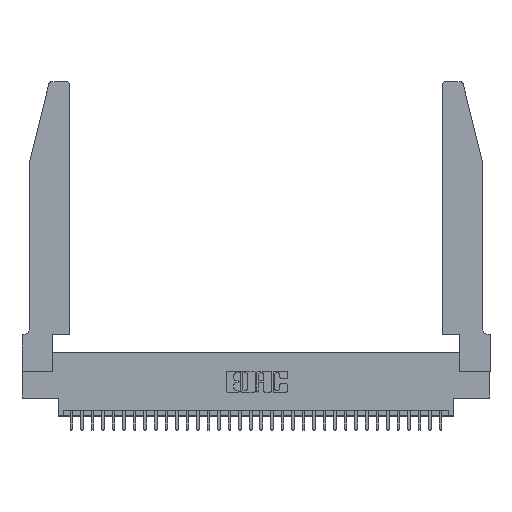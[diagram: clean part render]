
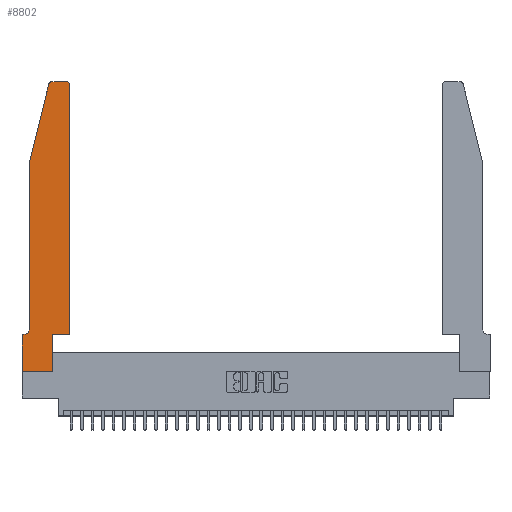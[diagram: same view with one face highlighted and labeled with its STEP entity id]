
A CAD part, top view. The second image highlights one B-rep face of the part: STEP entity #8802.
In plain terms, the highlighted planar face has unit normal (0, 0, 1).
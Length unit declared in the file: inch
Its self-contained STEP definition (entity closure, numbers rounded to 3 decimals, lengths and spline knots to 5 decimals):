
#25 = VERTEX_POINT ( 'NONE', #307 ) ;
#42 = CARTESIAN_POINT ( 'NONE',  ( 0.4505, 2.72, 0.37 ) ) ;
#307 = CARTESIAN_POINT ( 'NONE',  ( 0.0755, 0.42, 0.37 ) ) ;
#499 = CARTESIAN_POINT ( 'NONE',  ( 0.2865, 0.35, 0.37 ) ) ;
#1762 = VERTEX_POINT ( 'NONE', #8056 ) ;
#1792 = DIRECTION ( 'NONE',  ( 1., 0., 0. ) ) ;
#1813 = ORIENTED_EDGE ( 'NONE', *, *, #8376, .T. ) ;
#1943 = DIRECTION ( 'NONE',  ( 1., 0., 0. ) ) ;
#2092 = DIRECTION ( 'NONE',  ( 0., 0., -1. ) ) ;
#2441 = VECTOR ( 'NONE', #3148, 39.37008 ) ;
#2450 = DIRECTION ( 'NONE',  ( 1., 0., 0. ) ) ;
#2932 = LINE ( 'NONE', #30753, #23141 ) ;
#3148 = DIRECTION ( 'NONE',  ( 0., 1., 0. ) ) ;
#3216 = CARTESIAN_POINT ( 'NONE',  ( 0.4205, 2.75, 0.37 ) ) ;
#3739 = EDGE_CURVE ( 'NONE', #6368, #6413, #22148, .T. ) ;
#3926 = EDGE_CURVE ( 'NONE', #12568, #24901, #11070, .T. ) ;
#4892 = CARTESIAN_POINT ( 'NONE',  ( 0., 0., 0.37 ) ) ;
#4934 = VECTOR ( 'NONE', #24225, 39.37008 ) ;
#5141 = CARTESIAN_POINT ( 'NONE',  ( 0.4505, 0.35, 0.37 ) ) ;
#5718 = VERTEX_POINT ( 'NONE', #18212 ) ;
#6053 = DIRECTION ( 'NONE',  ( 0., -1., 0. ) ) ;
#6120 = ORIENTED_EDGE ( 'NONE', *, *, #23613, .T. ) ;
#6368 = VERTEX_POINT ( 'NONE', #12994 ) ;
#6413 = VERTEX_POINT ( 'NONE', #42 ) ;
#6601 = ORIENTED_EDGE ( 'NONE', *, *, #31092, .T. ) ;
#7410 = CARTESIAN_POINT ( 'NONE',  ( 0.0755, 0.35, 0.37 ) ) ;
#7532 = DIRECTION ( 'NONE',  ( -1., 0., 0. ) ) ;
#8056 = CARTESIAN_POINT ( 'NONE',  ( 0.0055, 0.35, 0.37 ) ) ;
#8376 = EDGE_CURVE ( 'NONE', #21702, #12568, #32842, .T. ) ;
#8802 = ADVANCED_FACE ( 'NONE', ( #28333 ), #31266, .T. ) ;
#9107 = ORIENTED_EDGE ( 'NONE', *, *, #26627, .T. ) ;
#9505 = CARTESIAN_POINT ( 'NONE',  ( 0., 0., 0.37 ) ) ;
#9605 = CARTESIAN_POINT ( 'NONE',  ( 0.284, 2.75, 0.37 ) ) ;
#10192 = EDGE_CURVE ( 'NONE', #20287, #16153, #25273, .T. ) ;
#10235 = LINE ( 'NONE', #4892, #24139 ) ;
#11070 = CIRCLE ( 'NONE', #30890, 0.03 ) ;
#11318 = CARTESIAN_POINT ( 'NONE',  ( 0.2605, 2.75, 0.37 ) ) ;
#12568 = VERTEX_POINT ( 'NONE', #9605 ) ;
#12684 = CIRCLE ( 'NONE', #32647, 0.07 ) ;
#12994 = CARTESIAN_POINT ( 'NONE',  ( 0.4505, 0.35, 0.37 ) ) ;
#13008 = EDGE_CURVE ( 'NONE', #5718, #25, #16957, .T. ) ;
#13115 = DIRECTION ( 'NONE',  ( 0., 1., 0. ) ) ;
#13818 = LINE ( 'NONE', #7410, #32206 ) ;
#14341 = VECTOR ( 'NONE', #13115, 39.37008 ) ;
#14389 = CARTESIAN_POINT ( 'NONE',  ( 0.284, 2.72, 0.37 ) ) ;
#14455 = EDGE_LOOP ( 'NONE', ( #1813, #28550, #6120, #15240, #16873, #18515, #21007, #15657, #6601, #9107, #24677, #20216 ) ) ;
#15134 = CIRCLE ( 'NONE', #17676, 0.03 ) ;
#15240 = ORIENTED_EDGE ( 'NONE', *, *, #13008, .T. ) ;
#15545 = CARTESIAN_POINT ( 'NONE',  ( 0., 0., 0.37 ) ) ;
#15585 = EDGE_CURVE ( 'NONE', #25, #1762, #12684, .T. ) ;
#15615 = CARTESIAN_POINT ( 'NONE',  ( 0., 0.35, 0.37 ) ) ;
#15657 = ORIENTED_EDGE ( 'NONE', *, *, #23441, .T. ) ;
#16100 = CARTESIAN_POINT ( 'NONE',  ( 0.0755, 2., 0.37 ) ) ;
#16153 = VERTEX_POINT ( 'NONE', #9505 ) ;
#16873 = ORIENTED_EDGE ( 'NONE', *, *, #15585, .T. ) ;
#16957 = LINE ( 'NONE', #19191, #23916 ) ;
#17021 = DIRECTION ( 'NONE',  ( 1., 0., 0. ) ) ;
#17129 = VERTEX_POINT ( 'NONE', #24206 ) ;
#17596 = DIRECTION ( 'NONE',  ( 0., 0., 1. ) ) ;
#17676 = AXIS2_PLACEMENT_3D ( 'NONE', #33218, #17596, #1792 ) ;
#17897 = CARTESIAN_POINT ( 'NONE',  ( 0.0055, 0.42, 0.37 ) ) ;
#18183 = DIRECTION ( 'NONE',  ( 0., -1., 0. ) ) ;
#18212 = CARTESIAN_POINT ( 'NONE',  ( 0.0755, 2., 0.37 ) ) ;
#18258 = DIRECTION ( 'NONE',  ( 0., 0., 1. ) ) ;
#18391 = LINE ( 'NONE', #16100, #31458 ) ;
#18515 = ORIENTED_EDGE ( 'NONE', *, *, #24323, .T. ) ;
#19191 = CARTESIAN_POINT ( 'NONE',  ( 0.0755, 2., 0.37 ) ) ;
#20216 = ORIENTED_EDGE ( 'NONE', *, *, #23313, .T. ) ;
#20287 = VERTEX_POINT ( 'NONE', #29115 ) ;
#20555 = DIRECTION ( 'NONE',  ( -1., 0., 0. ) ) ;
#21007 = ORIENTED_EDGE ( 'NONE', *, *, #10192, .T. ) ;
#21702 = VERTEX_POINT ( 'NONE', #3216 ) ;
#22148 = LINE ( 'NONE', #5141, #14341 ) ;
#23141 = VECTOR ( 'NONE', #1943, 39.37008 ) ;
#23313 = EDGE_CURVE ( 'NONE', #6413, #21702, #15134, .T. ) ;
#23330 = DIRECTION ( 'NONE',  ( 1., 0., 0. ) ) ;
#23441 = EDGE_CURVE ( 'NONE', #16153, #17129, #10235, .T. ) ;
#23457 = LINE ( 'NONE', #499, #2441 ) ;
#23613 = EDGE_CURVE ( 'NONE', #24901, #5718, #18391, .T. ) ;
#23916 = VECTOR ( 'NONE', #6053, 39.37008 ) ;
#24139 = VECTOR ( 'NONE', #23330, 39.37008 ) ;
#24206 = CARTESIAN_POINT ( 'NONE',  ( 0.2865, 0., 0.37 ) ) ;
#24225 = DIRECTION ( 'NONE',  ( -1., 0., 0. ) ) ;
#24323 = EDGE_CURVE ( 'NONE', #1762, #20287, #13818, .T. ) ;
#24677 = ORIENTED_EDGE ( 'NONE', *, *, #3739, .T. ) ;
#24901 = VERTEX_POINT ( 'NONE', #25476 ) ;
#25273 = LINE ( 'NONE', #15545, #31400 ) ;
#25476 = CARTESIAN_POINT ( 'NONE',  ( 0.25487, 2.72718, 0.37 ) ) ;
#25844 = CARTESIAN_POINT ( 'NONE',  ( 0.2865, 0.35, 0.37 ) ) ;
#26600 = DIRECTION ( 'NONE',  ( -0.239, -0.971, 0. ) ) ;
#26627 = EDGE_CURVE ( 'NONE', #30278, #6368, #2932, .T. ) ;
#28333 = FACE_OUTER_BOUND ( 'NONE', #14455, .T. ) ;
#28550 = ORIENTED_EDGE ( 'NONE', *, *, #3926, .T. ) ;
#29115 = CARTESIAN_POINT ( 'NONE',  ( 0., 0.35, 0.37 ) ) ;
#29242 = AXIS2_PLACEMENT_3D ( 'NONE', #15615, #18258, #2450 ) ;
#30278 = VERTEX_POINT ( 'NONE', #25844 ) ;
#30753 = CARTESIAN_POINT ( 'NONE',  ( 0.4505, 0.35, 0.37 ) ) ;
#30890 = AXIS2_PLACEMENT_3D ( 'NONE', #14389, #32649, #17021 ) ;
#31092 = EDGE_CURVE ( 'NONE', #17129, #30278, #23457, .T. ) ;
#31266 = PLANE ( 'NONE',  #29242 ) ;
#31400 = VECTOR ( 'NONE', #18183, 39.37008 ) ;
#31458 = VECTOR ( 'NONE', #26600, 39.37008 ) ;
#32206 = VECTOR ( 'NONE', #7532, 39.37008 ) ;
#32647 = AXIS2_PLACEMENT_3D ( 'NONE', #17897, #2092, #20555 ) ;
#32649 = DIRECTION ( 'NONE',  ( 0., 0., 1. ) ) ;
#32842 = LINE ( 'NONE', #11318, #4934 ) ;
#33218 = CARTESIAN_POINT ( 'NONE',  ( 0.4205, 2.72, 0.37 ) ) ;
